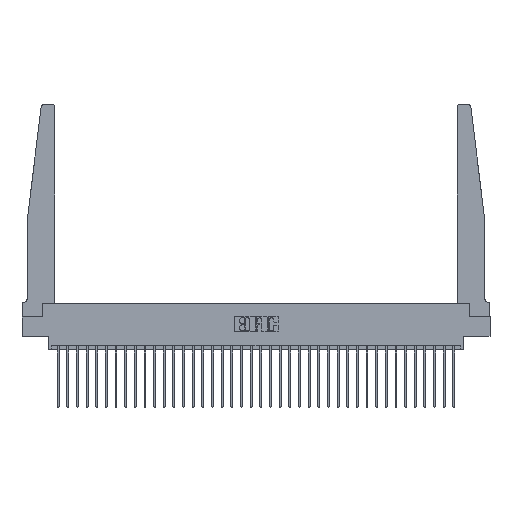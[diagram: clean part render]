
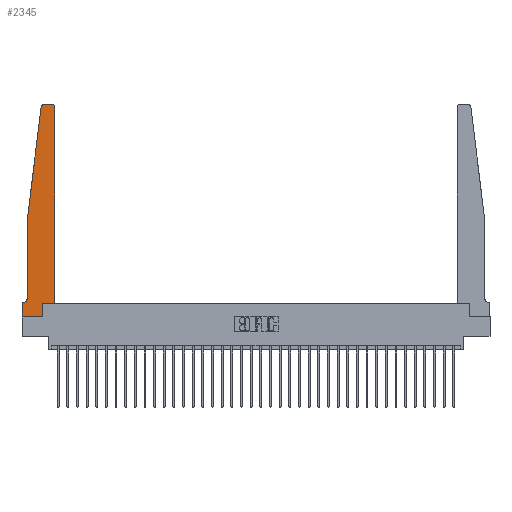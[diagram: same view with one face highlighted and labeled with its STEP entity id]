
A CAD part, top view. The second image highlights one B-rep face of the part: STEP entity #2345.
In plain terms, the highlighted planar face has unit normal (0, 0, 1).
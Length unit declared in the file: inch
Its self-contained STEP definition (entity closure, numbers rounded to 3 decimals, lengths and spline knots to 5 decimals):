
#58 = DIRECTION ( 'NONE',  ( 1., 0., 0. ) ) ;
#408 = DIRECTION ( 'NONE',  ( 1., 0., 0. ) ) ;
#624 = CARTESIAN_POINT ( 'NONE',  ( 0.425, 0.18, 0.37 ) ) ;
#1114 = CARTESIAN_POINT ( 'NONE',  ( 0.015, 0.1875, 0.37 ) ) ;
#1184 = CARTESIAN_POINT ( 'NONE',  ( 0.2605, 0.18, 0.37 ) ) ;
#1686 = VERTEX_POINT ( 'NONE', #24351 ) ;
#2011 = VECTOR ( 'NONE', #23640, 39.37008 ) ;
#2345 = ADVANCED_FACE ( 'NONE', ( #17392 ), #22047, .T. ) ;
#2737 = VECTOR ( 'NONE', #10459, 39.37008 ) ;
#3209 = LINE ( 'NONE', #624, #17200 ) ;
#3526 = EDGE_CURVE ( 'NONE', #28044, #9787, #17718, .T. ) ;
#4472 = CARTESIAN_POINT ( 'NONE',  ( 0.425, 0.18, 0.37 ) ) ;
#4800 = CARTESIAN_POINT ( 'NONE',  ( 0.2605, 0.18, 0.37 ) ) ;
#4995 = EDGE_CURVE ( 'NONE', #25637, #8622, #9406, .T. ) ;
#5152 = VERTEX_POINT ( 'NONE', #4472 ) ;
#5262 = CARTESIAN_POINT ( 'NONE',  ( 0.065, 1.25, 0.37 ) ) ;
#5841 = VERTEX_POINT ( 'NONE', #7234 ) ;
#6018 = AXIS2_PLACEMENT_3D ( 'NONE', #7114, #27044, #12116 ) ;
#6085 = EDGE_CURVE ( 'NONE', #22153, #30217, #27605, .T. ) ;
#6805 = CARTESIAN_POINT ( 'NONE',  ( 0., 0.1875, 0.37 ) ) ;
#7114 = CARTESIAN_POINT ( 'NONE',  ( 0., 0.1875, 0.37 ) ) ;
#7177 = DIRECTION ( 'NONE',  ( 0., 0., 1. ) ) ;
#7234 = CARTESIAN_POINT ( 'NONE',  ( 0., 0., 0.37 ) ) ;
#7373 = VERTEX_POINT ( 'NONE', #29298 ) ;
#7563 = ORIENTED_EDGE ( 'NONE', *, *, #15295, .T. ) ;
#8208 = CARTESIAN_POINT ( 'NONE',  ( 0.25, 2.75, 0.37 ) ) ;
#8555 = ORIENTED_EDGE ( 'NONE', *, *, #4995, .T. ) ;
#8594 = EDGE_CURVE ( 'NONE', #9979, #22153, #16133, .T. ) ;
#8622 = VERTEX_POINT ( 'NONE', #4800 ) ;
#8839 = ORIENTED_EDGE ( 'NONE', *, *, #24458, .T. ) ;
#9293 = DIRECTION ( 'NONE',  ( -0.122, -0.992, 0. ) ) ;
#9406 = LINE ( 'NONE', #1184, #2011 ) ;
#9787 = VERTEX_POINT ( 'NONE', #6805 ) ;
#9979 = VERTEX_POINT ( 'NONE', #28540 ) ;
#10164 = DIRECTION ( 'NONE',  ( 0., -1., 0. ) ) ;
#10459 = DIRECTION ( 'NONE',  ( 1., 0., 0. ) ) ;
#10781 = LINE ( 'NONE', #15606, #24023 ) ;
#10785 = VERTEX_POINT ( 'NONE', #5262 ) ;
#11375 = ORIENTED_EDGE ( 'NONE', *, *, #6085, .T. ) ;
#11635 = LINE ( 'NONE', #11701, #16701 ) ;
#11701 = CARTESIAN_POINT ( 'NONE',  ( 0.065, 1.25, 0.37 ) ) ;
#11765 = ORIENTED_EDGE ( 'NONE', *, *, #13122, .T. ) ;
#12116 = DIRECTION ( 'NONE',  ( 1., 0., 0. ) ) ;
#12631 = EDGE_CURVE ( 'NONE', #8622, #5152, #19866, .T. ) ;
#12710 = CIRCLE ( 'NONE', #24363, 0.03 ) ;
#12963 = CARTESIAN_POINT ( 'NONE',  ( 0., 0., 0.37 ) ) ;
#13122 = EDGE_CURVE ( 'NONE', #1686, #10785, #11635, .T. ) ;
#13458 = ORIENTED_EDGE ( 'NONE', *, *, #19621, .T. ) ;
#13762 = DIRECTION ( 'NONE',  ( 0., 0., -1. ) ) ;
#13766 = CARTESIAN_POINT ( 'NONE',  ( 0.27653, 2.75, 0.37 ) ) ;
#15295 = EDGE_CURVE ( 'NONE', #9787, #5841, #10781, .T. ) ;
#15352 = DIRECTION ( 'NONE',  ( 0., 0., 1. ) ) ;
#15597 = CIRCLE ( 'NONE', #30355, 0.05 ) ;
#15606 = CARTESIAN_POINT ( 'NONE',  ( 0., 0., 0.37 ) ) ;
#15946 = AXIS2_PLACEMENT_3D ( 'NONE', #22106, #7177, #24592 ) ;
#15965 = LINE ( 'NONE', #12963, #2737 ) ;
#16133 = CIRCLE ( 'NONE', #15946, 0.03 ) ;
#16253 = ORIENTED_EDGE ( 'NONE', *, *, #25805, .T. ) ;
#16701 = VECTOR ( 'NONE', #9293, 39.37008 ) ;
#16910 = VECTOR ( 'NONE', #21975, 39.37008 ) ;
#17200 = VECTOR ( 'NONE', #18072, 39.37008 ) ;
#17392 = FACE_OUTER_BOUND ( 'NONE', #18041, .T. ) ;
#17521 = VECTOR ( 'NONE', #58, 39.37008 ) ;
#17718 = LINE ( 'NONE', #24356, #16910 ) ;
#18041 = EDGE_LOOP ( 'NONE', ( #11375, #16253, #11765, #8839, #30504, #29399, #7563, #13458, #8555, #29637, #26895, #28182 ) ) ;
#18072 = DIRECTION ( 'NONE',  ( 0., 1., 0. ) ) ;
#18234 = EDGE_CURVE ( 'NONE', #5152, #9979, #3209, .T. ) ;
#19621 = EDGE_CURVE ( 'NONE', #5841, #25637, #15965, .T. ) ;
#19866 = LINE ( 'NONE', #29991, #17521 ) ;
#20611 = DIRECTION ( 'NONE',  ( -1., 0., 0. ) ) ;
#21180 = VECTOR ( 'NONE', #24667, 39.37008 ) ;
#21975 = DIRECTION ( 'NONE',  ( -1., 0., 0. ) ) ;
#22047 = PLANE ( 'NONE',  #6018 ) ;
#22106 = CARTESIAN_POINT ( 'NONE',  ( 0.395, 2.72, 0.37 ) ) ;
#22110 = CARTESIAN_POINT ( 'NONE',  ( 0.2605, 0., 0.37 ) ) ;
#22153 = VERTEX_POINT ( 'NONE', #24619 ) ;
#23640 = DIRECTION ( 'NONE',  ( 0., 1., 0. ) ) ;
#24023 = VECTOR ( 'NONE', #10164, 39.37008 ) ;
#24351 = CARTESIAN_POINT ( 'NONE',  ( 0.24675, 2.72367, 0.37 ) ) ;
#24356 = CARTESIAN_POINT ( 'NONE',  ( 0.065, 0.1875, 0.37 ) ) ;
#24363 = AXIS2_PLACEMENT_3D ( 'NONE', #30330, #15352, #408 ) ;
#24458 = EDGE_CURVE ( 'NONE', #10785, #7373, #27805, .T. ) ;
#24592 = DIRECTION ( 'NONE',  ( 1., 0., 0. ) ) ;
#24619 = CARTESIAN_POINT ( 'NONE',  ( 0.395, 2.75, 0.37 ) ) ;
#24667 = DIRECTION ( 'NONE',  ( 0., -1., 0. ) ) ;
#25637 = VERTEX_POINT ( 'NONE', #22110 ) ;
#25805 = EDGE_CURVE ( 'NONE', #30217, #1686, #12710, .T. ) ;
#26809 = VECTOR ( 'NONE', #20611, 39.37008 ) ;
#26895 = ORIENTED_EDGE ( 'NONE', *, *, #18234, .T. ) ;
#27044 = DIRECTION ( 'NONE',  ( 0., 0., 1. ) ) ;
#27173 = CARTESIAN_POINT ( 'NONE',  ( 0.065, 1.25, 0.37 ) ) ;
#27605 = LINE ( 'NONE', #8208, #26809 ) ;
#27805 = LINE ( 'NONE', #27173, #21180 ) ;
#28044 = VERTEX_POINT ( 'NONE', #1114 ) ;
#28182 = ORIENTED_EDGE ( 'NONE', *, *, #8594, .T. ) ;
#28540 = CARTESIAN_POINT ( 'NONE',  ( 0.425, 2.72, 0.37 ) ) ;
#28728 = CARTESIAN_POINT ( 'NONE',  ( 0.015, 0.2375, 0.37 ) ) ;
#29298 = CARTESIAN_POINT ( 'NONE',  ( 0.065, 0.2375, 0.37 ) ) ;
#29399 = ORIENTED_EDGE ( 'NONE', *, *, #3526, .T. ) ;
#29637 = ORIENTED_EDGE ( 'NONE', *, *, #12631, .T. ) ;
#29991 = CARTESIAN_POINT ( 'NONE',  ( 0.425, 0.18, 0.37 ) ) ;
#30217 = VERTEX_POINT ( 'NONE', #13766 ) ;
#30328 = EDGE_CURVE ( 'NONE', #7373, #28044, #15597, .T. ) ;
#30330 = CARTESIAN_POINT ( 'NONE',  ( 0.27653, 2.72, 0.37 ) ) ;
#30355 = AXIS2_PLACEMENT_3D ( 'NONE', #28728, #13762, #31260 ) ;
#30504 = ORIENTED_EDGE ( 'NONE', *, *, #30328, .T. ) ;
#31260 = DIRECTION ( 'NONE',  ( -1., 0., 0. ) ) ;
